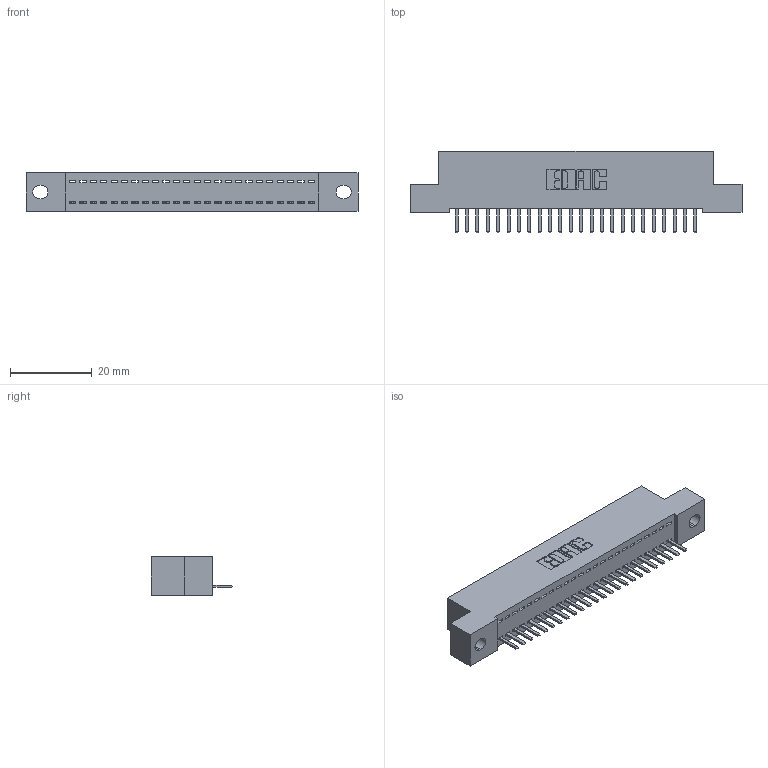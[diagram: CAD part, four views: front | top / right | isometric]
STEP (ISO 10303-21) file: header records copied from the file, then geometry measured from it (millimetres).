
FILE_DESCRIPTION (( 'STEP AP203' ), '1' );
FILE_NAME ('392-024-520-102.STEP', '2019-10-07T07:04:26', ( '' ), ( '' ), 'SwSTEP 2.0', 'SolidWorks 2016', '' );
FILE_SCHEMA (( 'CONFIG_CONTROL_DESIGN' ));
Length unit declared in the file: inch
Products named in the file (3): 345-292-001_345-293-120; 392-024-520-102; 342 Part_.128 Slot
Assembly tree (25 placements, depth 2):
  392-024-520-102
    342 Part_.128 Slot
    345-292-001_345-293-120  x24
Bounding box: 81.28 x 20.02 x 9.4 mm (x, y, z)
Volume: 6939.1 mm3; surface area: 9392.6 mm2
Topology: 25 solids, 25 shells, 1602 faces, 4727 edges, 3086 vertices
Faces by surface type: plane 1126, cylinder 476
Entity records: 17117 total; most frequent: CARTESIAN_POINT 2974, ORIENTED_EDGE 2922, DIRECTION 2533, EDGE_CURVE 1461, VECTOR 1329, LINE 1329, VERTEX_POINT 970, AXIS2_PLACEMENT_3D 602
